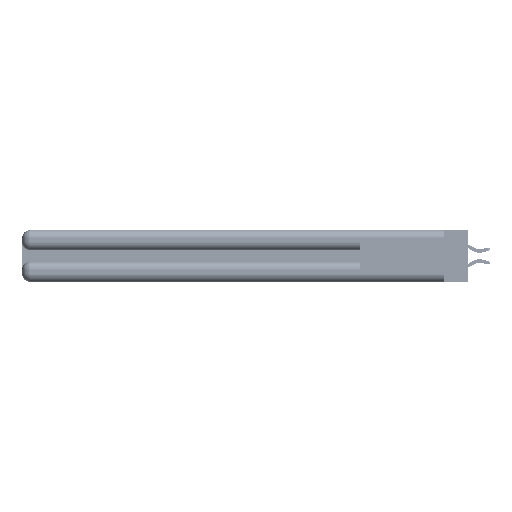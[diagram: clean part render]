
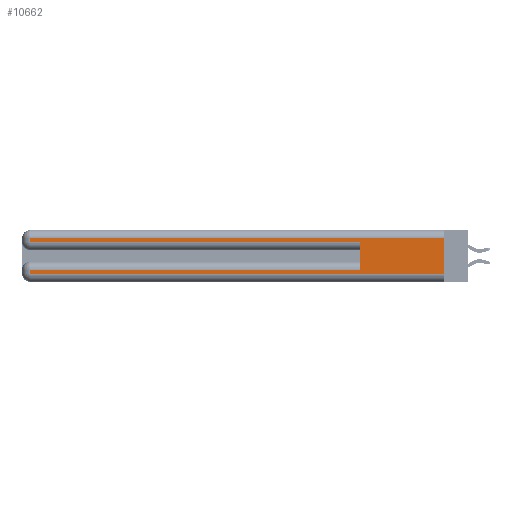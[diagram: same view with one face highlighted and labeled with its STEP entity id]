
A CAD part, left-side view. The second image highlights one B-rep face of the part: STEP entity #10662.
In plain terms, the highlighted planar face has unit normal (-1, 0, 0).
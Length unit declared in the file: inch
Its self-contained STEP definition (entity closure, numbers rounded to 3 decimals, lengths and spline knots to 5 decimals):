
#1176 = VECTOR ( 'NONE', #14304, 39.37008 ) ;
#2195 = VECTOR ( 'NONE', #36753, 39.37008 ) ;
#2588 = ORIENTED_EDGE ( 'NONE', *, *, #38219, .F. ) ;
#5024 = ORIENTED_EDGE ( 'NONE', *, *, #39189, .T. ) ;
#7619 = DIRECTION ( 'NONE',  ( 0., 1., 0. ) ) ;
#8102 = ORIENTED_EDGE ( 'NONE', *, *, #44542, .T. ) ;
#8862 = CARTESIAN_POINT ( 'NONE',  ( 0., 0., 0.37 ) ) ;
#10259 = ORIENTED_EDGE ( 'NONE', *, *, #25257, .F. ) ;
#10483 = LINE ( 'NONE', #42403, #11070 ) ;
#10662 = ADVANCED_FACE ( 'NONE', ( #36524 ), #19148, .F. ) ;
#10805 = EDGE_CURVE ( 'NONE', #36879, #12511, #39524, .T. ) ;
#11070 = VECTOR ( 'NONE', #15107, 39.37008 ) ;
#12282 = EDGE_LOOP ( 'NONE', ( #2588, #8102, #41540, #19681, #10259, #36957, #49589, #5024 ) ) ;
#12511 = VERTEX_POINT ( 'NONE', #15359 ) ;
#13069 = CARTESIAN_POINT ( 'NONE',  ( 0., 0., 0.06 ) ) ;
#13173 = CARTESIAN_POINT ( 'NONE',  ( 0., 0., 0.31 ) ) ;
#13431 = VECTOR ( 'NONE', #35814, 39.37008 ) ;
#14304 = DIRECTION ( 'NONE',  ( 0., -1., 0. ) ) ;
#14798 = EDGE_CURVE ( 'NONE', #36191, #21709, #16926, .T. ) ;
#15107 = DIRECTION ( 'NONE',  ( 0., 0., -1. ) ) ;
#15359 = CARTESIAN_POINT ( 'NONE',  ( 0., 2.94, 0.085 ) ) ;
#16905 = CARTESIAN_POINT ( 'NONE',  ( 0., 2.94, 0.06 ) ) ;
#16926 = LINE ( 'NONE', #42090, #1176 ) ;
#19148 = PLANE ( 'NONE',  #24484 ) ;
#19681 = ORIENTED_EDGE ( 'NONE', *, *, #14798, .T. ) ;
#19974 = CARTESIAN_POINT ( 'NONE',  ( 0., 0., 0.085 ) ) ;
#20367 = LINE ( 'NONE', #8862, #47684 ) ;
#20501 = VERTEX_POINT ( 'NONE', #13173 ) ;
#20992 = LINE ( 'NONE', #32201, #2195 ) ;
#21709 = VERTEX_POINT ( 'NONE', #37905 ) ;
#22838 = DIRECTION ( 'NONE',  ( 1., 0., 0. ) ) ;
#23006 = DIRECTION ( 'NONE',  ( 0., 0., -1. ) ) ;
#23915 = VERTEX_POINT ( 'NONE', #13069 ) ;
#24322 = LINE ( 'NONE', #40687, #37687 ) ;
#24484 = AXIS2_PLACEMENT_3D ( 'NONE', #46267, #22838, #23006 ) ;
#25257 = EDGE_CURVE ( 'NONE', #36879, #21709, #20992, .T. ) ;
#27073 = VERTEX_POINT ( 'NONE', #16905 ) ;
#27283 = CARTESIAN_POINT ( 'NONE',  ( 0., 0., 0.31 ) ) ;
#27378 = VECTOR ( 'NONE', #27592, 39.37008 ) ;
#27592 = DIRECTION ( 'NONE',  ( 0., 1., 0. ) ) ;
#27888 = EDGE_CURVE ( 'NONE', #12511, #27073, #10483, .T. ) ;
#28921 = CARTESIAN_POINT ( 'NONE',  ( 0., 2.94, 0.31 ) ) ;
#31038 = LINE ( 'NONE', #31917, #13431 ) ;
#31917 = CARTESIAN_POINT ( 'NONE',  ( 0., 0., 0.06 ) ) ;
#31970 = DIRECTION ( 'NONE',  ( 0., 0., -1. ) ) ;
#32201 = CARTESIAN_POINT ( 'NONE',  ( 0., 0.6, 0.145 ) ) ;
#32304 = VERTEX_POINT ( 'NONE', #28921 ) ;
#34474 = CARTESIAN_POINT ( 'NONE',  ( 0., 0.6, 0.085 ) ) ;
#34828 = LINE ( 'NONE', #27283, #45111 ) ;
#35814 = DIRECTION ( 'NONE',  ( 0., -1., 0. ) ) ;
#36191 = VERTEX_POINT ( 'NONE', #38062 ) ;
#36308 = DIRECTION ( 'NONE',  ( 0., 0., -1. ) ) ;
#36524 = FACE_OUTER_BOUND ( 'NONE', #12282, .T. ) ;
#36753 = DIRECTION ( 'NONE',  ( 0., 0., 1. ) ) ;
#36879 = VERTEX_POINT ( 'NONE', #34474 ) ;
#36957 = ORIENTED_EDGE ( 'NONE', *, *, #10805, .T. ) ;
#37687 = VECTOR ( 'NONE', #36308, 39.37008 ) ;
#37905 = CARTESIAN_POINT ( 'NONE',  ( 0., 0.6, 0.285 ) ) ;
#38062 = CARTESIAN_POINT ( 'NONE',  ( 0., 2.94, 0.285 ) ) ;
#38219 = EDGE_CURVE ( 'NONE', #20501, #23915, #20367, .T. ) ;
#39189 = EDGE_CURVE ( 'NONE', #27073, #23915, #31038, .T. ) ;
#39524 = LINE ( 'NONE', #19974, #27378 ) ;
#40687 = CARTESIAN_POINT ( 'NONE',  ( 0., 2.94, 0.37 ) ) ;
#41540 = ORIENTED_EDGE ( 'NONE', *, *, #48479, .T. ) ;
#42090 = CARTESIAN_POINT ( 'NONE',  ( 0., 0., 0.285 ) ) ;
#42403 = CARTESIAN_POINT ( 'NONE',  ( 0., 2.94, 0.37 ) ) ;
#44542 = EDGE_CURVE ( 'NONE', #20501, #32304, #34828, .T. ) ;
#45111 = VECTOR ( 'NONE', #7619, 39.37008 ) ;
#46267 = CARTESIAN_POINT ( 'NONE',  ( 0., 0., 0.37 ) ) ;
#47684 = VECTOR ( 'NONE', #31970, 39.37008 ) ;
#48479 = EDGE_CURVE ( 'NONE', #32304, #36191, #24322, .T. ) ;
#49589 = ORIENTED_EDGE ( 'NONE', *, *, #27888, .T. ) ;
